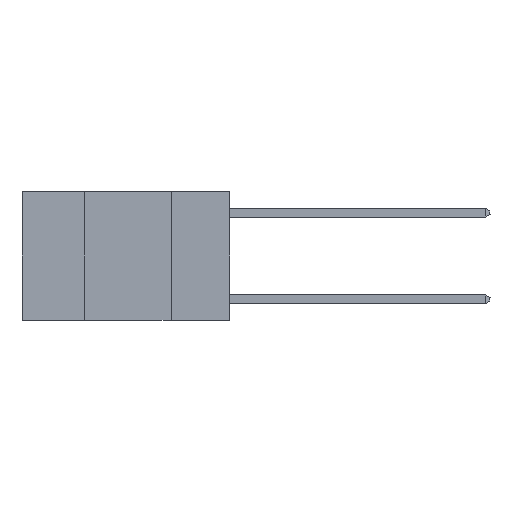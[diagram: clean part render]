
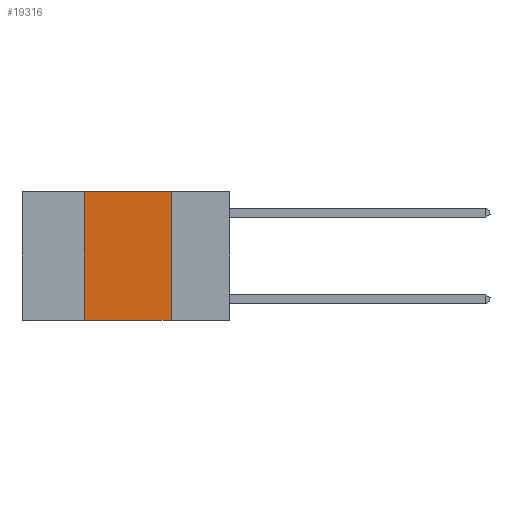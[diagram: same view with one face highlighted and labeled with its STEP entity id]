
A CAD part, left-side view. The second image highlights one B-rep face of the part: STEP entity #19316.
In plain terms, the highlighted planar face has unit normal (-1, 0, 0).
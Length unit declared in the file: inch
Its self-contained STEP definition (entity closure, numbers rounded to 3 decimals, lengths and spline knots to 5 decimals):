
#136 = VERTEX_POINT ( 'NONE', #10805 ) ;
#578 = CARTESIAN_POINT ( 'NONE',  ( 0., 0.17, -0.37 ) ) ;
#1508 = VERTEX_POINT ( 'NONE', #18424 ) ;
#2508 = LINE ( 'NONE', #14339, #16216 ) ;
#3784 = EDGE_CURVE ( 'NONE', #1508, #20868, #14527, .T. ) ;
#4727 = CARTESIAN_POINT ( 'NONE',  ( 0., 0.6, -0.37 ) ) ;
#5823 = DIRECTION ( 'NONE',  ( 0., 0., -1. ) ) ;
#8961 = VERTEX_POINT ( 'NONE', #16997 ) ;
#10805 = CARTESIAN_POINT ( 'NONE',  ( 0., 0.17, 0. ) ) ;
#11030 = VECTOR ( 'NONE', #24308, 39.37008 ) ;
#11717 = CARTESIAN_POINT ( 'NONE',  ( 0., 0.17, 0. ) ) ;
#14339 = CARTESIAN_POINT ( 'NONE',  ( 0., 0.42, 0. ) ) ;
#14527 = LINE ( 'NONE', #4727, #11030 ) ;
#14795 = LINE ( 'NONE', #22661, #19688 ) ;
#14933 = VECTOR ( 'NONE', #5823, 39.37008 ) ;
#15763 = DIRECTION ( 'NONE',  ( 1., 0., 0. ) ) ;
#15881 = PLANE ( 'NONE',  #21793 ) ;
#16216 = VECTOR ( 'NONE', #22197, 39.37008 ) ;
#16830 = ORIENTED_EDGE ( 'NONE', *, *, #3784, .T. ) ;
#16997 = CARTESIAN_POINT ( 'NONE',  ( 0., 0.42, 0. ) ) ;
#18059 = DIRECTION ( 'NONE',  ( 0., 0., -1. ) ) ;
#18424 = CARTESIAN_POINT ( 'NONE',  ( 0., 0.42, -0.37 ) ) ;
#19084 = LINE ( 'NONE', #11717, #14933 ) ;
#19316 = ADVANCED_FACE ( 'NONE', ( #23732 ), #15881, .F. ) ;
#19688 = VECTOR ( 'NONE', #22396, 39.37008 ) ;
#20520 = ORIENTED_EDGE ( 'NONE', *, *, #22495, .F. ) ;
#20868 = VERTEX_POINT ( 'NONE', #578 ) ;
#21539 = ORIENTED_EDGE ( 'NONE', *, *, #24521, .F. ) ;
#21793 = AXIS2_PLACEMENT_3D ( 'NONE', #21795, #15763, #18059 ) ;
#21795 = CARTESIAN_POINT ( 'NONE',  ( 0., 0.6, 0. ) ) ;
#22197 = DIRECTION ( 'NONE',  ( 0., 0., 1. ) ) ;
#22396 = DIRECTION ( 'NONE',  ( 0., -1., 0. ) ) ;
#22495 = EDGE_CURVE ( 'NONE', #136, #20868, #19084, .T. ) ;
#22661 = CARTESIAN_POINT ( 'NONE',  ( 0., 0.6, 0. ) ) ;
#22847 = ORIENTED_EDGE ( 'NONE', *, *, #23655, .F. ) ;
#23242 = EDGE_LOOP ( 'NONE', ( #20520, #21539, #22847, #16830 ) ) ;
#23655 = EDGE_CURVE ( 'NONE', #1508, #8961, #2508, .T. ) ;
#23732 = FACE_OUTER_BOUND ( 'NONE', #23242, .T. ) ;
#24308 = DIRECTION ( 'NONE',  ( 0., -1., 0. ) ) ;
#24521 = EDGE_CURVE ( 'NONE', #8961, #136, #14795, .T. ) ;
